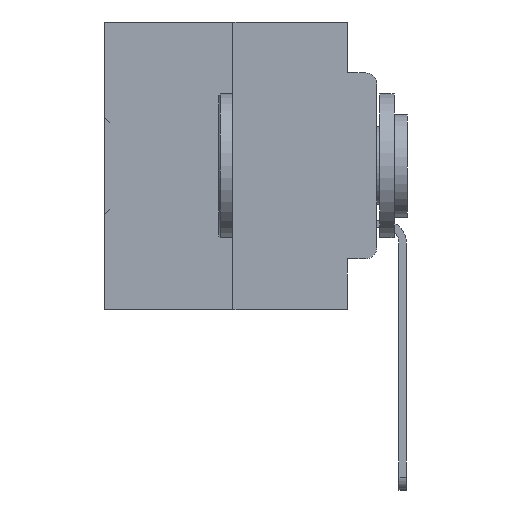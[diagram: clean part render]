
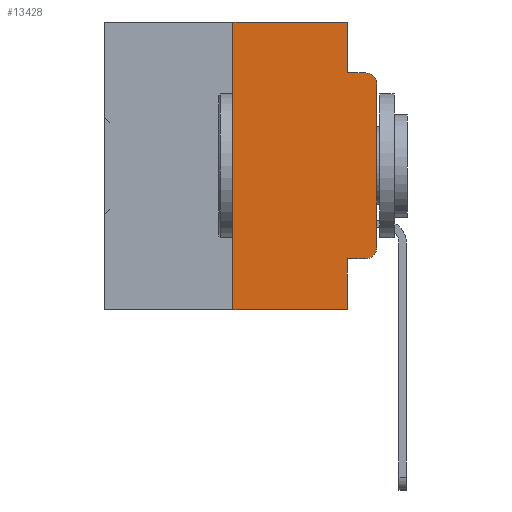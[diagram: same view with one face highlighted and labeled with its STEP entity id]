
A CAD part, left-side view. The second image highlights one B-rep face of the part: STEP entity #13428.
In plain terms, the highlighted planar face has unit normal (-1, 0, 0).
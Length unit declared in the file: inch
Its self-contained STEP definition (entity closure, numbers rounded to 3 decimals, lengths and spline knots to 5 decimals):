
#27 = VERTEX_POINT ( 'NONE', #16819 ) ;
#180 = ORIENTED_EDGE ( 'NONE', *, *, #16709, .T. ) ;
#809 = CARTESIAN_POINT ( 'NONE',  ( 0., 0.25, -0.5 ) ) ;
#962 = DIRECTION ( 'NONE',  ( 0., 0., -1. ) ) ;
#2043 = CARTESIAN_POINT ( 'NONE',  ( 0., 0.051, -0.0885 ) ) ;
#2110 = CARTESIAN_POINT ( 'NONE',  ( 0., 0.051, 0. ) ) ;
#2218 = EDGE_LOOP ( 'NONE', ( #7508, #180, #16574, #18465, #33857, #28098, #5125, #36541, #22239, #38294 ) ) ;
#2281 = LINE ( 'NONE', #33306, #9503 ) ;
#2995 = DIRECTION ( 'NONE',  ( 0., -1., 0. ) ) ;
#3229 = CARTESIAN_POINT ( 'NONE',  ( 0., 0.473, 0. ) ) ;
#3905 = LINE ( 'NONE', #9011, #33621 ) ;
#4521 = VERTEX_POINT ( 'NONE', #12570 ) ;
#4974 = CARTESIAN_POINT ( 'NONE',  ( 0., 0.051, 0. ) ) ;
#5039 = EDGE_CURVE ( 'NONE', #19229, #31394, #3905, .T. ) ;
#5125 = ORIENTED_EDGE ( 'NONE', *, *, #26725, .T. ) ;
#5831 = CIRCLE ( 'NONE', #13707, 0.02 ) ;
#5893 = LINE ( 'NONE', #2110, #13038 ) ;
#6727 = LINE ( 'NONE', #22520, #21912 ) ;
#7508 = ORIENTED_EDGE ( 'NONE', *, *, #27320, .T. ) ;
#7556 = AXIS2_PLACEMENT_3D ( 'NONE', #10277, #30933, #13303 ) ;
#8313 = VERTEX_POINT ( 'NONE', #26154 ) ;
#9011 = CARTESIAN_POINT ( 'NONE',  ( 0., 0.051, -0.4115 ) ) ;
#9115 = VERTEX_POINT ( 'NONE', #809 ) ;
#9116 = EDGE_CURVE ( 'NONE', #31394, #8313, #5831, .T. ) ;
#9253 = VECTOR ( 'NONE', #17548, 39.37008 ) ;
#9302 = CARTESIAN_POINT ( 'NONE',  ( 0., 0.02, -0.4115 ) ) ;
#9503 = VECTOR ( 'NONE', #15864, 39.37008 ) ;
#10277 = CARTESIAN_POINT ( 'NONE',  ( 0., 0.02, -0.1085 ) ) ;
#11389 = DIRECTION ( 'NONE',  ( 0., -1., 0. ) ) ;
#11402 = DIRECTION ( 'NONE',  ( 0., 0., -1. ) ) ;
#12570 = CARTESIAN_POINT ( 'NONE',  ( 0., 0.051, 0. ) ) ;
#13038 = VECTOR ( 'NONE', #11402, 39.37008 ) ;
#13303 = DIRECTION ( 'NONE',  ( 0., 0., -1. ) ) ;
#13428 = ADVANCED_FACE ( 'NONE', ( #19934 ), #30140, .F. ) ;
#13707 = AXIS2_PLACEMENT_3D ( 'NONE', #36575, #19341, #962 ) ;
#15520 = DIRECTION ( 'NONE',  ( 0., 0., -1. ) ) ;
#15864 = DIRECTION ( 'NONE',  ( 0., 0., 1. ) ) ;
#16175 = LINE ( 'NONE', #4974, #23201 ) ;
#16574 = ORIENTED_EDGE ( 'NONE', *, *, #28646, .F. ) ;
#16704 = VECTOR ( 'NONE', #23182, 39.37008 ) ;
#16709 = EDGE_CURVE ( 'NONE', #27, #19643, #36050, .T. ) ;
#16819 = CARTESIAN_POINT ( 'NONE',  ( 0., 0., -0.1085 ) ) ;
#17548 = DIRECTION ( 'NONE',  ( 0., 0., 1. ) ) ;
#18465 = ORIENTED_EDGE ( 'NONE', *, *, #30317, .F. ) ;
#19229 = VERTEX_POINT ( 'NONE', #24565 ) ;
#19341 = DIRECTION ( 'NONE',  ( -1., 0., 0. ) ) ;
#19643 = VERTEX_POINT ( 'NONE', #35359 ) ;
#19934 = FACE_OUTER_BOUND ( 'NONE', #2218, .T. ) ;
#19983 = CARTESIAN_POINT ( 'NONE',  ( 0., 0.25, 0. ) ) ;
#20073 = VECTOR ( 'NONE', #11389, 39.37008 ) ;
#21912 = VECTOR ( 'NONE', #28308, 39.37008 ) ;
#22239 = ORIENTED_EDGE ( 'NONE', *, *, #5039, .T. ) ;
#22520 = CARTESIAN_POINT ( 'NONE',  ( 0., 0.473, 0. ) ) ;
#23182 = DIRECTION ( 'NONE',  ( 0., -1., 0. ) ) ;
#23201 = VECTOR ( 'NONE', #25895, 39.37008 ) ;
#23308 = EDGE_CURVE ( 'NONE', #9115, #37855, #2281, .T. ) ;
#24565 = CARTESIAN_POINT ( 'NONE',  ( 0., 0.051, -0.4115 ) ) ;
#25895 = DIRECTION ( 'NONE',  ( 0., 0., -1. ) ) ;
#26154 = CARTESIAN_POINT ( 'NONE',  ( 0., 0., -0.3915 ) ) ;
#26396 = EDGE_CURVE ( 'NONE', #37855, #4521, #6727, .T. ) ;
#26725 = EDGE_CURVE ( 'NONE', #9115, #28696, #33089, .T. ) ;
#27320 = EDGE_CURVE ( 'NONE', #8313, #27, #32815, .T. ) ;
#27831 = LINE ( 'NONE', #37560, #20073 ) ;
#28098 = ORIENTED_EDGE ( 'NONE', *, *, #23308, .F. ) ;
#28308 = DIRECTION ( 'NONE',  ( 0., -1., 0. ) ) ;
#28646 = EDGE_CURVE ( 'NONE', #29448, #19643, #27831, .T. ) ;
#28696 = VERTEX_POINT ( 'NONE', #29262 ) ;
#29262 = CARTESIAN_POINT ( 'NONE',  ( 0., 0.051, -0.5 ) ) ;
#29412 = AXIS2_PLACEMENT_3D ( 'NONE', #3229, #32994, #15520 ) ;
#29448 = VERTEX_POINT ( 'NONE', #2043 ) ;
#30140 = PLANE ( 'NONE',  #29412 ) ;
#30317 = EDGE_CURVE ( 'NONE', #4521, #29448, #16175, .T. ) ;
#30933 = DIRECTION ( 'NONE',  ( -1., 0., 0. ) ) ;
#31394 = VERTEX_POINT ( 'NONE', #9302 ) ;
#32017 = CARTESIAN_POINT ( 'NONE',  ( 0., 0., 0. ) ) ;
#32815 = LINE ( 'NONE', #32017, #9253 ) ;
#32994 = DIRECTION ( 'NONE',  ( 1., 0., 0. ) ) ;
#33089 = LINE ( 'NONE', #37389, #16704 ) ;
#33306 = CARTESIAN_POINT ( 'NONE',  ( 0., 0.25, 0. ) ) ;
#33621 = VECTOR ( 'NONE', #2995, 39.37008 ) ;
#33857 = ORIENTED_EDGE ( 'NONE', *, *, #26396, .F. ) ;
#34779 = EDGE_CURVE ( 'NONE', #19229, #28696, #5893, .T. ) ;
#35359 = CARTESIAN_POINT ( 'NONE',  ( 0., 0.02, -0.0885 ) ) ;
#36050 = CIRCLE ( 'NONE', #7556, 0.02 ) ;
#36541 = ORIENTED_EDGE ( 'NONE', *, *, #34779, .F. ) ;
#36575 = CARTESIAN_POINT ( 'NONE',  ( 0., 0.02, -0.3915 ) ) ;
#37389 = CARTESIAN_POINT ( 'NONE',  ( 0., 0.473, -0.5 ) ) ;
#37560 = CARTESIAN_POINT ( 'NONE',  ( 0., 0.051, -0.0885 ) ) ;
#37855 = VERTEX_POINT ( 'NONE', #19983 ) ;
#38294 = ORIENTED_EDGE ( 'NONE', *, *, #9116, .T. ) ;
